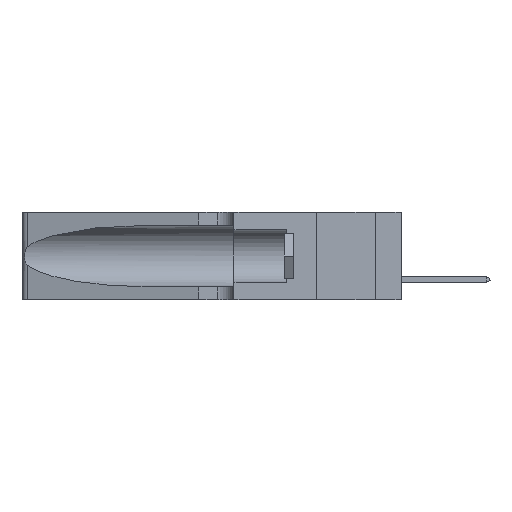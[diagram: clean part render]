
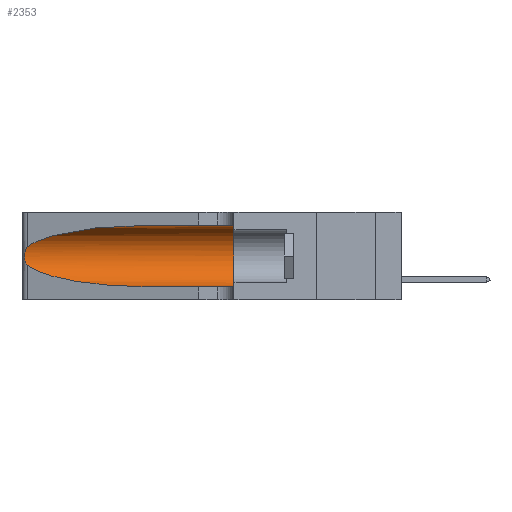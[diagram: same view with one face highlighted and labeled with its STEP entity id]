
A CAD part, left-side view. The second image highlights one B-rep face of the part: STEP entity #2353.
In plain terms, the highlighted cylindrical face has radius 3.308 mm (diameter 6.617 mm), a partial arc.
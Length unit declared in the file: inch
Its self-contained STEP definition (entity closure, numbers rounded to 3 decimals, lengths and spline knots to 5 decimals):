
#156 = CARTESIAN_POINT ( 'NONE',  ( 0.25639, 1.23184, 0.21858 ) ) ;
#169 = VECTOR ( 'NONE', #24259, 39.37008 ) ;
#985 = CARTESIAN_POINT ( 'NONE',  ( 0.25487, 1.22718, 0.14631 ) ) ;
#2058 = EDGE_LOOP ( 'NONE', ( #16585, #12906, #17074, #21118, #25660, #8769 ) ) ;
#2353 = ADVANCED_FACE ( 'NONE', ( #21423 ), #12887, .F. ) ;
#2511 = VERTEX_POINT ( 'NONE', #12702 ) ;
#2675 = CARTESIAN_POINT ( 'NONE',  ( 0.25487, 1.22718, 0.14631 ) ) ;
#3078 = CARTESIAN_POINT ( 'NONE',  ( 0.26075, 1.23896, 0.178 ) ) ;
#3293 = VERTEX_POINT ( 'NONE', #19543 ) ;
#3759 = EDGE_CURVE ( 'NONE', #19208, #10520, #29201, .T. ) ;
#4055 = DIRECTION ( 'NONE',  ( 0., 1., 0. ) ) ;
#4630 = CARTESIAN_POINT ( 'NONE',  ( 0.25487, 1.22718, 0.22369 ) ) ;
#5390 = CARTESIAN_POINT ( 'NONE',  ( 0.25789, 1.23486, 0.15765 ) ) ;
#5815 = EDGE_CURVE ( 'NONE', #8121, #19208, #14409, .T. ) ;
#6991 = EDGE_CURVE ( 'NONE', #13337, #2511, #18028, .T. ) ;
#7215 = CARTESIAN_POINT ( 'NONE',  ( 0.1305, 1.61858, 0.185 ) ) ;
#7623 = CARTESIAN_POINT ( 'NONE',  ( 0.25487, 1.22718, 0.14631 ) ) ;
#7877 = CARTESIAN_POINT ( 'NONE',  ( 0.25639, 1.23186, 0.15144 ) ) ;
#8083 = CARTESIAN_POINT ( 'NONE',  ( 0.25487, 1.22718, 0.22369 ) ) ;
#8121 = VERTEX_POINT ( 'NONE', #17566 ) ;
#8615 = CARTESIAN_POINT ( 'NONE',  ( 0.2373, 1.15595, 0.08982 ) ) ;
#8769 = ORIENTED_EDGE ( 'NONE', *, *, #25990, .F. ) ;
#8799 = CARTESIAN_POINT ( 'NONE',  ( 0.2373, 1.15595, 0.28018 ) ) ;
#9146 = CARTESIAN_POINT ( 'NONE',  ( 0.1305, 1.61858, 0.31525 ) ) ;
#9723 = DIRECTION ( 'NONE',  ( 0., -1., 0. ) ) ;
#9944 = LINE ( 'NONE', #9146, #18039 ) ;
#10520 = VERTEX_POINT ( 'NONE', #7623 ) ;
#11030 = CARTESIAN_POINT ( 'NONE',  ( 0.25487, 1.22718, 0.22369 ) ) ;
#11547 = DIRECTION ( 'NONE',  ( 0., 0., 1. ) ) ;
#11662 = CARTESIAN_POINT ( 'NONE',  ( 0.1305, 0.72297, 0.05475 ) ) ;
#12007 =( BOUNDED_CURVE ( )  B_SPLINE_CURVE ( 3, ( #985, #8615, #21387, #11662 ),
 .UNSPECIFIED., .F., .T. ) 
 B_SPLINE_CURVE_WITH_KNOTS ( ( 4, 4 ),
 ( 3.44316, 4.71239 ),
 .UNSPECIFIED. ) 
 CURVE ( )  GEOMETRIC_REPRESENTATION_ITEM ( )  RATIONAL_B_SPLINE_CURVE ( ( 1., 0.87, 0.87, 1. ) ) 
 REPRESENTATION_ITEM ( '' )  );
#12702 = CARTESIAN_POINT ( 'NONE',  ( 0.1305, 0.35, 0.05475 ) ) ;
#12780 = CARTESIAN_POINT ( 'NONE',  ( 0.26075, 1.23896, 0.19203 ) ) ;
#12887 = CYLINDRICAL_SURFACE ( 'NONE', #26416, 0.13025 ) ;
#12906 = ORIENTED_EDGE ( 'NONE', *, *, #3759, .T. ) ;
#13337 = VERTEX_POINT ( 'NONE', #28199 ) ;
#14409 =( BOUNDED_CURVE ( )  B_SPLINE_CURVE ( 3, ( #18985, #30181, #8799, #11030 ),
 .UNSPECIFIED., .F., .F. ) 
 B_SPLINE_CURVE_WITH_KNOTS ( ( 4, 4 ),
 ( 1.5708, 2.84003 ),
 .UNSPECIFIED. ) 
 CURVE ( )  GEOMETRIC_REPRESENTATION_ITEM ( )  RATIONAL_B_SPLINE_CURVE ( ( 1., 0.87, 0.87, 1. ) ) 
 REPRESENTATION_ITEM ( '' )  );
#15285 = DIRECTION ( 'NONE',  ( 0., -1., 0. ) ) ;
#15359 = CARTESIAN_POINT ( 'NONE',  ( 0.25854, 1.2359, 0.20912 ) ) ;
#16402 = CARTESIAN_POINT ( 'NONE',  ( 0.1305, 0.35, 0.185 ) ) ;
#16585 = ORIENTED_EDGE ( 'NONE', *, *, #5815, .T. ) ;
#17074 = ORIENTED_EDGE ( 'NONE', *, *, #28133, .T. ) ;
#17566 = CARTESIAN_POINT ( 'NONE',  ( 0.1305, 0.72297, 0.31525 ) ) ;
#17732 = CARTESIAN_POINT ( 'NONE',  ( 0.25856, 1.23593, 0.16098 ) ) ;
#17936 = CARTESIAN_POINT ( 'NONE',  ( 0.26018, 1.23835, 0.19895 ) ) ;
#18028 = LINE ( 'NONE', #31565, #169 ) ;
#18039 = VECTOR ( 'NONE', #15285, 39.37008 ) ;
#18855 = EDGE_CURVE ( 'NONE', #3293, #2511, #23795, .T. ) ;
#18985 = CARTESIAN_POINT ( 'NONE',  ( 0.1305, 0.72297, 0.31525 ) ) ;
#19208 = VERTEX_POINT ( 'NONE', #4630 ) ;
#19543 = CARTESIAN_POINT ( 'NONE',  ( 0.1305, 0.35, 0.31525 ) ) ;
#20422 = CARTESIAN_POINT ( 'NONE',  ( 0.25555, 1.22993, 0.14849 ) ) ;
#21118 = ORIENTED_EDGE ( 'NONE', *, *, #6991, .T. ) ;
#21387 = CARTESIAN_POINT ( 'NONE',  ( 0.18966, 0.96281, 0.05475 ) ) ;
#21423 = FACE_OUTER_BOUND ( 'NONE', #2058, .T. ) ;
#23795 = CIRCLE ( 'NONE', #27935, 0.13025 ) ;
#24259 = DIRECTION ( 'NONE',  ( 0., -1., 0. ) ) ;
#25399 = CARTESIAN_POINT ( 'NONE',  ( 0.26017, 1.23833, 0.17102 ) ) ;
#25660 = ORIENTED_EDGE ( 'NONE', *, *, #18855, .F. ) ;
#25990 = EDGE_CURVE ( 'NONE', #8121, #3293, #9944, .T. ) ;
#26416 = AXIS2_PLACEMENT_3D ( 'NONE', #7215, #9723, #26990 ) ;
#26990 = DIRECTION ( 'NONE',  ( 0., 0., -1. ) ) ;
#27536 = CARTESIAN_POINT ( 'NONE',  ( 0.25555, 1.22994, 0.2215 ) ) ;
#27935 = AXIS2_PLACEMENT_3D ( 'NONE', #16402, #4055, #11547 ) ;
#28133 = EDGE_CURVE ( 'NONE', #10520, #13337, #12007, .T. ) ;
#28199 = CARTESIAN_POINT ( 'NONE',  ( 0.1305, 0.72297, 0.05475 ) ) ;
#29201 = B_SPLINE_CURVE_WITH_KNOTS ( 'NONE', 3,
 ( #8083, #27536, #156, #30233, #15359, #17936, #12780, #3078, #25399, #17732, #5390, #7877, #20422, #2675 ),
 .UNSPECIFIED., .F., .F.,
 ( 4, 2, 2, 2, 2, 2, 4 ),
 ( 0., 0.00027, 0.00053, 0.00107, 0.0016, 0.00187, 0.00214 ),
 .UNSPECIFIED. ) ;
#30181 = CARTESIAN_POINT ( 'NONE',  ( 0.18966, 0.96281, 0.31525 ) ) ;
#30233 = CARTESIAN_POINT ( 'NONE',  ( 0.25787, 1.23484, 0.2124 ) ) ;
#31565 = CARTESIAN_POINT ( 'NONE',  ( 0.1305, 1.61858, 0.05475 ) ) ;
